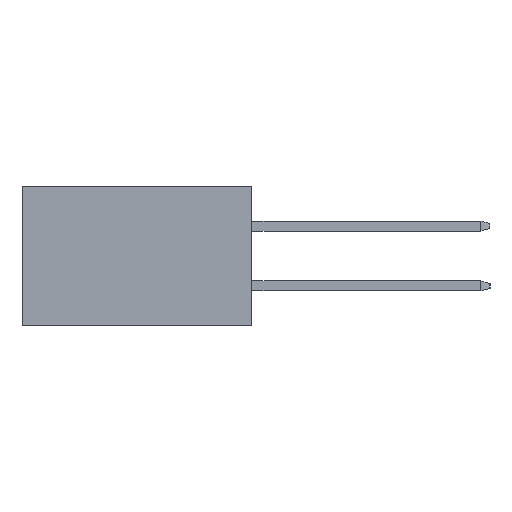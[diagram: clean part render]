
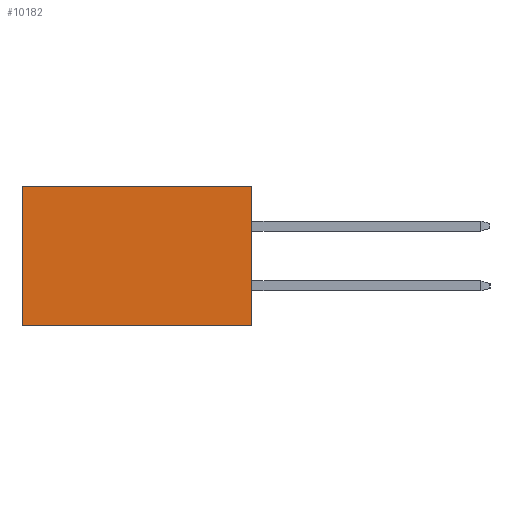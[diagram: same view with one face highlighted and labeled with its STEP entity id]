
A CAD part, left-side view. The second image highlights one B-rep face of the part: STEP entity #10182.
In plain terms, the highlighted planar face has unit normal (-1, 0, 0).
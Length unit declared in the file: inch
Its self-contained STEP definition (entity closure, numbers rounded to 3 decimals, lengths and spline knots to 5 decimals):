
#150 = EDGE_CURVE ( 'NONE', #15256, #16519, #16367, .T. ) ;
#193 = ORIENTED_EDGE ( 'NONE', *, *, #8597, .T. ) ;
#495 = VECTOR ( 'NONE', #10595, 39.37008 ) ;
#1108 = ORIENTED_EDGE ( 'NONE', *, *, #5731, .F. ) ;
#1129 = LINE ( 'NONE', #9134, #495 ) ;
#3560 = CARTESIAN_POINT ( 'NONE',  ( 0.3205, 0., -0.437 ) ) ;
#4738 = CARTESIAN_POINT ( 'NONE',  ( 0.3205, 0., -0.437 ) ) ;
#5015 = LINE ( 'NONE', #4738, #12352 ) ;
#5058 = DIRECTION ( 'NONE',  ( 0., 1., 0. ) ) ;
#5457 = PLANE ( 'NONE',  #7076 ) ;
#5535 = FACE_OUTER_BOUND ( 'NONE', #10003, .T. ) ;
#5731 = EDGE_CURVE ( 'NONE', #16519, #13834, #5015, .T. ) ;
#6360 = EDGE_CURVE ( 'NONE', #9435, #13834, #1129, .T. ) ;
#7076 = AXIS2_PLACEMENT_3D ( 'NONE', #16769, #15424, #8231 ) ;
#7480 = VECTOR ( 'NONE', #9339, 39.37008 ) ;
#7596 = ORIENTED_EDGE ( 'NONE', *, *, #150, .F. ) ;
#7725 = DIRECTION ( 'NONE',  ( 0., 1., 0. ) ) ;
#7845 = ORIENTED_EDGE ( 'NONE', *, *, #6360, .T. ) ;
#8231 = DIRECTION ( 'NONE',  ( 0., 0., -1. ) ) ;
#8597 = EDGE_CURVE ( 'NONE', #15256, #9435, #10566, .T. ) ;
#9134 = CARTESIAN_POINT ( 'NONE',  ( 0.3205, 0.72, -0.437 ) ) ;
#9339 = DIRECTION ( 'NONE',  ( 0., 0., -1. ) ) ;
#9435 = VERTEX_POINT ( 'NONE', #16814 ) ;
#10003 = EDGE_LOOP ( 'NONE', ( #7845, #1108, #7596, #193 ) ) ;
#10182 = ADVANCED_FACE ( 'NONE', ( #5535 ), #5457, .F. ) ;
#10391 = CARTESIAN_POINT ( 'NONE',  ( 0.3205, 0., 0. ) ) ;
#10566 = LINE ( 'NONE', #10391, #17100 ) ;
#10595 = DIRECTION ( 'NONE',  ( 0., 0., -1. ) ) ;
#12352 = VECTOR ( 'NONE', #7725, 39.37008 ) ;
#13834 = VERTEX_POINT ( 'NONE', #15837 ) ;
#15256 = VERTEX_POINT ( 'NONE', #16239 ) ;
#15424 = DIRECTION ( 'NONE',  ( 1., 0., 0. ) ) ;
#15837 = CARTESIAN_POINT ( 'NONE',  ( 0.3205, 0.72, -0.437 ) ) ;
#16239 = CARTESIAN_POINT ( 'NONE',  ( 0.3205, 0., 0. ) ) ;
#16367 = LINE ( 'NONE', #17364, #7480 ) ;
#16519 = VERTEX_POINT ( 'NONE', #3560 ) ;
#16769 = CARTESIAN_POINT ( 'NONE',  ( 0.3205, 0., -0.437 ) ) ;
#16814 = CARTESIAN_POINT ( 'NONE',  ( 0.3205, 0.72, 0. ) ) ;
#17100 = VECTOR ( 'NONE', #5058, 39.37008 ) ;
#17364 = CARTESIAN_POINT ( 'NONE',  ( 0.3205, 0., -0.437 ) ) ;
